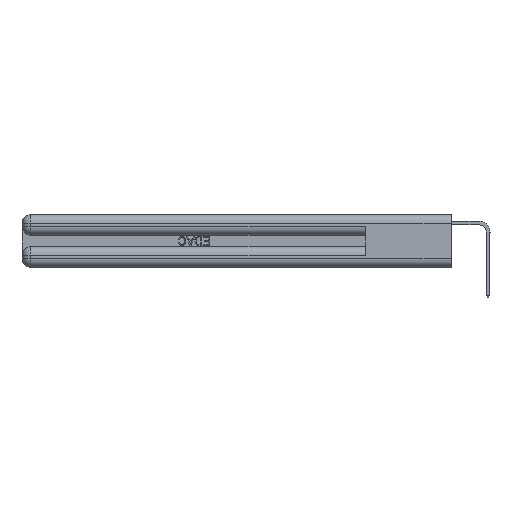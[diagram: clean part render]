
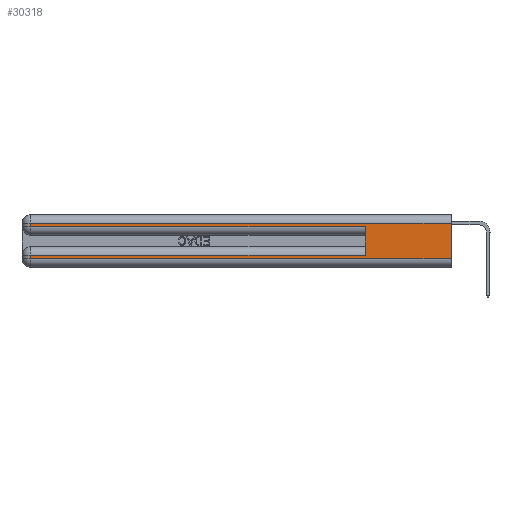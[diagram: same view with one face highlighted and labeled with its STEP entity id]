
A CAD part, left-side view. The second image highlights one B-rep face of the part: STEP entity #30318.
In plain terms, the highlighted planar face has unit normal (-1, 0, 0).
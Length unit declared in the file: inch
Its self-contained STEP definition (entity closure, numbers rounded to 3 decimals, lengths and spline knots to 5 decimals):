
#80 = VERTEX_POINT ( 'NONE', #15162 ) ;
#146 = LINE ( 'NONE', #19969, #18438 ) ;
#366 = DIRECTION ( 'NONE',  ( 0., -1., 0. ) ) ;
#374 = EDGE_CURVE ( 'NONE', #7023, #23493, #28271, .T. ) ;
#499 = FACE_OUTER_BOUND ( 'NONE', #11889, .T. ) ;
#1009 = DIRECTION ( 'NONE',  ( 0., 1., 0. ) ) ;
#1792 = CARTESIAN_POINT ( 'NONE',  ( 0., 2.94, 0.37 ) ) ;
#2032 = LINE ( 'NONE', #24839, #26605 ) ;
#2120 = DIRECTION ( 'NONE',  ( 0., 0., -1. ) ) ;
#3006 = EDGE_CURVE ( 'NONE', #7165, #80, #26908, .T. ) ;
#4192 = ORIENTED_EDGE ( 'NONE', *, *, #8175, .T. ) ;
#4201 = CARTESIAN_POINT ( 'NONE',  ( 0., 2.94, 0.085 ) ) ;
#4748 = LINE ( 'NONE', #1792, #23021 ) ;
#4790 = CARTESIAN_POINT ( 'NONE',  ( 0., 2.94, 0.31 ) ) ;
#5215 = ORIENTED_EDGE ( 'NONE', *, *, #3006, .F. ) ;
#6330 = LINE ( 'NONE', #16733, #29366 ) ;
#7023 = VERTEX_POINT ( 'NONE', #4790 ) ;
#7165 = VERTEX_POINT ( 'NONE', #12563 ) ;
#7335 = DIRECTION ( 'NONE',  ( 0., 0., -1. ) ) ;
#7351 = CARTESIAN_POINT ( 'NONE',  ( 0., 0.6, 0.085 ) ) ;
#8175 = EDGE_CURVE ( 'NONE', #12373, #10731, #6330, .T. ) ;
#9119 = DIRECTION ( 'NONE',  ( 0., 0., -1. ) ) ;
#9250 = PLANE ( 'NONE',  #12992 ) ;
#10731 = VERTEX_POINT ( 'NONE', #4201 ) ;
#11428 = EDGE_CURVE ( 'NONE', #12373, #21853, #2032, .T. ) ;
#11578 = CARTESIAN_POINT ( 'NONE',  ( 0., 2.94, 0.285 ) ) ;
#11889 = EDGE_LOOP ( 'NONE', ( #5215, #20813, #13348, #26823, #13240, #4192, #16698, #24678 ) ) ;
#11980 = DIRECTION ( 'NONE',  ( 0., 1., 0. ) ) ;
#12103 = VERTEX_POINT ( 'NONE', #29917 ) ;
#12188 = CARTESIAN_POINT ( 'NONE',  ( 0., 0., 0.37 ) ) ;
#12343 = CARTESIAN_POINT ( 'NONE',  ( 0., 0., 0.06 ) ) ;
#12373 = VERTEX_POINT ( 'NONE', #7351 ) ;
#12563 = CARTESIAN_POINT ( 'NONE',  ( 0., 0., 0.31 ) ) ;
#12992 = AXIS2_PLACEMENT_3D ( 'NONE', #30628, #16442, #2120 ) ;
#13240 = ORIENTED_EDGE ( 'NONE', *, *, #11428, .F. ) ;
#13270 = EDGE_CURVE ( 'NONE', #7165, #7023, #20179, .T. ) ;
#13348 = ORIENTED_EDGE ( 'NONE', *, *, #374, .T. ) ;
#13946 = VECTOR ( 'NONE', #1009, 39.37008 ) ;
#15162 = CARTESIAN_POINT ( 'NONE',  ( 0., 0., 0.06 ) ) ;
#15462 = DIRECTION ( 'NONE',  ( 0., 0., 1. ) ) ;
#15519 = LINE ( 'NONE', #12343, #26602 ) ;
#15605 = EDGE_CURVE ( 'NONE', #23493, #21853, #146, .T. ) ;
#15708 = VECTOR ( 'NONE', #25569, 39.37008 ) ;
#16442 = DIRECTION ( 'NONE',  ( 1., 0., 0. ) ) ;
#16698 = ORIENTED_EDGE ( 'NONE', *, *, #19503, .T. ) ;
#16733 = CARTESIAN_POINT ( 'NONE',  ( 0., 0., 0.085 ) ) ;
#17610 = DIRECTION ( 'NONE',  ( 0., -1., 0. ) ) ;
#18438 = VECTOR ( 'NONE', #17610, 39.37008 ) ;
#19503 = EDGE_CURVE ( 'NONE', #10731, #12103, #4748, .T. ) ;
#19969 = CARTESIAN_POINT ( 'NONE',  ( 0., 0., 0.285 ) ) ;
#20179 = LINE ( 'NONE', #22387, #13946 ) ;
#20813 = ORIENTED_EDGE ( 'NONE', *, *, #13270, .T. ) ;
#21853 = VERTEX_POINT ( 'NONE', #26538 ) ;
#22387 = CARTESIAN_POINT ( 'NONE',  ( 0., 0., 0.31 ) ) ;
#23021 = VECTOR ( 'NONE', #9119, 39.37008 ) ;
#23493 = VERTEX_POINT ( 'NONE', #11578 ) ;
#23954 = VECTOR ( 'NONE', #7335, 39.37008 ) ;
#24678 = ORIENTED_EDGE ( 'NONE', *, *, #29827, .T. ) ;
#24839 = CARTESIAN_POINT ( 'NONE',  ( 0., 0.6, 0.145 ) ) ;
#25569 = DIRECTION ( 'NONE',  ( 0., 0., -1. ) ) ;
#25667 = CARTESIAN_POINT ( 'NONE',  ( 0., 2.94, 0.37 ) ) ;
#26538 = CARTESIAN_POINT ( 'NONE',  ( 0., 0.6, 0.285 ) ) ;
#26602 = VECTOR ( 'NONE', #366, 39.37008 ) ;
#26605 = VECTOR ( 'NONE', #15462, 39.37008 ) ;
#26823 = ORIENTED_EDGE ( 'NONE', *, *, #15605, .T. ) ;
#26908 = LINE ( 'NONE', #12188, #23954 ) ;
#28271 = LINE ( 'NONE', #25667, #15708 ) ;
#29366 = VECTOR ( 'NONE', #11980, 39.37008 ) ;
#29827 = EDGE_CURVE ( 'NONE', #12103, #80, #15519, .T. ) ;
#29917 = CARTESIAN_POINT ( 'NONE',  ( 0., 2.94, 0.06 ) ) ;
#30318 = ADVANCED_FACE ( 'NONE', ( #499 ), #9250, .F. ) ;
#30628 = CARTESIAN_POINT ( 'NONE',  ( 0., 0., 0.37 ) ) ;
